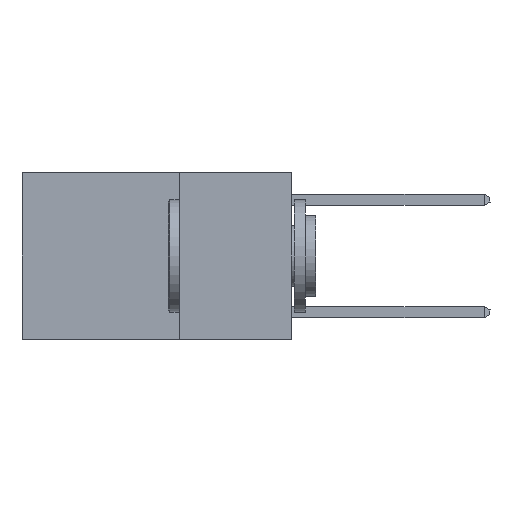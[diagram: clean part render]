
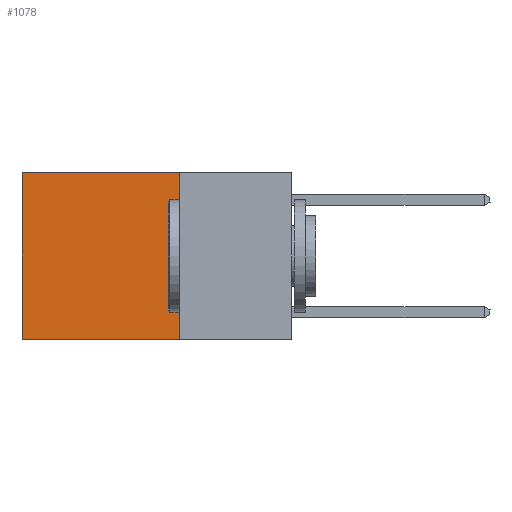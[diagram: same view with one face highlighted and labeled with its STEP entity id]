
A CAD part, left-side view. The second image highlights one B-rep face of the part: STEP entity #1078.
In plain terms, the highlighted planar face has unit normal (-1, 0, 0).
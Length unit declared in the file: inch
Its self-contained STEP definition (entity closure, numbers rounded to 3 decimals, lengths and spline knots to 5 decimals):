
#968 = LINE ( 'NONE', #14543, #16833 ) ;
#1078 = ADVANCED_FACE ( 'NONE', ( #19144 ), #19727, .F. ) ;
#3559 = DIRECTION ( 'NONE',  ( 0., 0., -1. ) ) ;
#3668 = EDGE_CURVE ( 'NONE', #19207, #9996, #5255, .T. ) ;
#4161 = VERTEX_POINT ( 'NONE', #19401 ) ;
#5255 = LINE ( 'NONE', #6101, #20484 ) ;
#5540 = ORIENTED_EDGE ( 'NONE', *, *, #26492, .T. ) ;
#6101 = CARTESIAN_POINT ( 'NONE',  ( 0.2625, 0.25, 0. ) ) ;
#7454 = CARTESIAN_POINT ( 'NONE',  ( 0.2625, 0.6, -0.37 ) ) ;
#7897 = EDGE_CURVE ( 'NONE', #19207, #4161, #26446, .T. ) ;
#8104 = DIRECTION ( 'NONE',  ( 1., 0., 0. ) ) ;
#8282 = VECTOR ( 'NONE', #27039, 39.37008 ) ;
#9110 = DIRECTION ( 'NONE',  ( 0., 1., 0. ) ) ;
#9547 = CARTESIAN_POINT ( 'NONE',  ( 0.2625, 0.25, -0.37 ) ) ;
#9647 = DIRECTION ( 'NONE',  ( 0., 0., -1. ) ) ;
#9996 = VERTEX_POINT ( 'NONE', #9547 ) ;
#10093 = DIRECTION ( 'NONE',  ( 0., 0., -1. ) ) ;
#12476 = ORIENTED_EDGE ( 'NONE', *, *, #7897, .T. ) ;
#13985 = EDGE_CURVE ( 'NONE', #9996, #14166, #15707, .T. ) ;
#14166 = VERTEX_POINT ( 'NONE', #7454 ) ;
#14543 = CARTESIAN_POINT ( 'NONE',  ( 0.2625, 0.6, 0. ) ) ;
#15707 = LINE ( 'NONE', #27419, #23785 ) ;
#16308 = AXIS2_PLACEMENT_3D ( 'NONE', #24410, #8104, #3559 ) ;
#16833 = VECTOR ( 'NONE', #10093, 39.37008 ) ;
#19144 = FACE_OUTER_BOUND ( 'NONE', #24755, .T. ) ;
#19207 = VERTEX_POINT ( 'NONE', #25253 ) ;
#19401 = CARTESIAN_POINT ( 'NONE',  ( 0.2625, 0.6, 0. ) ) ;
#19727 = PLANE ( 'NONE',  #16308 ) ;
#20484 = VECTOR ( 'NONE', #9647, 39.37008 ) ;
#21571 = CARTESIAN_POINT ( 'NONE',  ( 0.2625, 0.25, 0. ) ) ;
#23785 = VECTOR ( 'NONE', #9110, 39.37008 ) ;
#24410 = CARTESIAN_POINT ( 'NONE',  ( 0.2625, 0.25, 0. ) ) ;
#24755 = EDGE_LOOP ( 'NONE', ( #5540, #26489, #27369, #12476 ) ) ;
#25253 = CARTESIAN_POINT ( 'NONE',  ( 0.2625, 0.25, 0. ) ) ;
#26446 = LINE ( 'NONE', #21571, #8282 ) ;
#26489 = ORIENTED_EDGE ( 'NONE', *, *, #13985, .F. ) ;
#26492 = EDGE_CURVE ( 'NONE', #4161, #14166, #968, .T. ) ;
#27039 = DIRECTION ( 'NONE',  ( 0., 1., 0. ) ) ;
#27369 = ORIENTED_EDGE ( 'NONE', *, *, #3668, .F. ) ;
#27419 = CARTESIAN_POINT ( 'NONE',  ( 0.2625, 0.25, -0.37 ) ) ;
